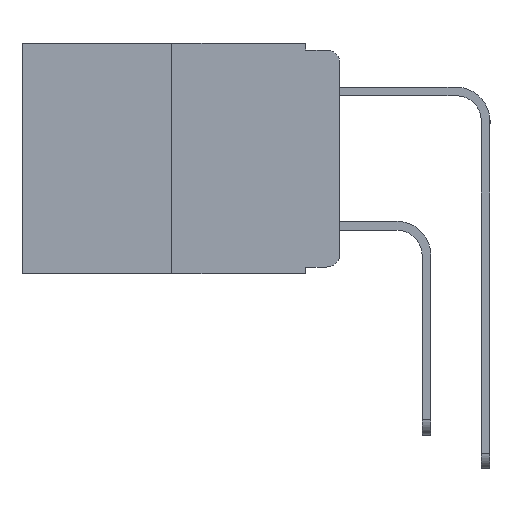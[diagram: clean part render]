
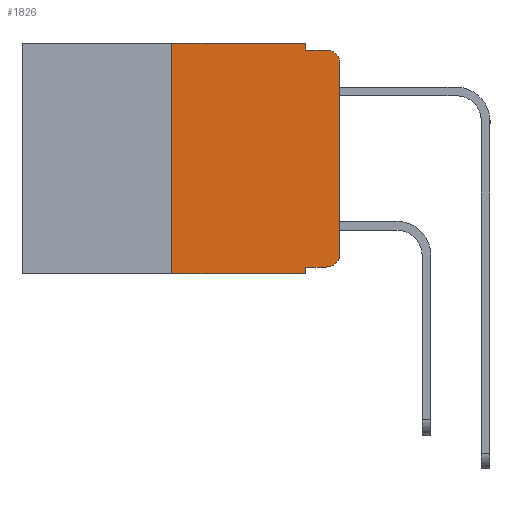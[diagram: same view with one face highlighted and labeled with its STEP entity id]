
A CAD part, left-side view. The second image highlights one B-rep face of the part: STEP entity #1826.
In plain terms, the highlighted planar face has unit normal (-1, 0, 0).
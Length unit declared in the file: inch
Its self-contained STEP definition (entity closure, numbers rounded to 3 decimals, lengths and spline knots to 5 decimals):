
#178 = FACE_OUTER_BOUND ( 'NONE', #17588, .T. ) ;
#365 = DIRECTION ( 'NONE',  ( 0., -1., 0. ) ) ;
#547 = VERTEX_POINT ( 'NONE', #4173 ) ;
#1144 = DIRECTION ( 'NONE',  ( 0., -1., 0. ) ) ;
#1159 = CARTESIAN_POINT ( 'NONE',  ( 0., 0., 0. ) ) ;
#1238 = EDGE_CURVE ( 'NONE', #547, #10272, #10835, .T. ) ;
#1810 = AXIS2_PLACEMENT_3D ( 'NONE', #14146, #5944, #15483 ) ;
#1826 = ADVANCED_FACE ( 'NONE', ( #178 ), #17150, .F. ) ;
#2052 = LINE ( 'NONE', #4103, #12909 ) ;
#3402 = DIRECTION ( 'NONE',  ( 0., 0., -1. ) ) ;
#3408 = VERTEX_POINT ( 'NONE', #6793 ) ;
#3584 = VERTEX_POINT ( 'NONE', #5995 ) ;
#3617 = EDGE_CURVE ( 'NONE', #3408, #16759, #14103, .T. ) ;
#3671 = ORIENTED_EDGE ( 'NONE', *, *, #1238, .F. ) ;
#3751 = AXIS2_PLACEMENT_3D ( 'NONE', #17131, #18101, #16671 ) ;
#3930 = AXIS2_PLACEMENT_3D ( 'NONE', #8382, #17770, #9779 ) ;
#4103 = CARTESIAN_POINT ( 'NONE',  ( 0., 0.051, 0. ) ) ;
#4173 = CARTESIAN_POINT ( 'NONE',  ( 0., 0.051, -0.01 ) ) ;
#4498 = DIRECTION ( 'NONE',  ( 0., -1., 0. ) ) ;
#4552 = VERTEX_POINT ( 'NONE', #11109 ) ;
#4815 = CARTESIAN_POINT ( 'NONE',  ( 0., 0.051, -0.01 ) ) ;
#4975 = CARTESIAN_POINT ( 'NONE',  ( 0., 0.051, -0.333 ) ) ;
#5243 = EDGE_CURVE ( 'NONE', #13959, #10272, #8101, .T. ) ;
#5551 = LINE ( 'NONE', #9230, #15588 ) ;
#5595 = DIRECTION ( 'NONE',  ( 0., 0., -1. ) ) ;
#5944 = DIRECTION ( 'NONE',  ( -1., 0., 0. ) ) ;
#5995 = CARTESIAN_POINT ( 'NONE',  ( 0., 0.25, 0. ) ) ;
#6417 = VECTOR ( 'NONE', #1144, 39.37008 ) ;
#6580 = ORIENTED_EDGE ( 'NONE', *, *, #5243, .T. ) ;
#6598 = ORIENTED_EDGE ( 'NONE', *, *, #8454, .T. ) ;
#6631 = ORIENTED_EDGE ( 'NONE', *, *, #10300, .T. ) ;
#6708 = VECTOR ( 'NONE', #4498, 39.37008 ) ;
#6731 = LINE ( 'NONE', #15886, #11270 ) ;
#6792 = DIRECTION ( 'NONE',  ( 0., 0., 1. ) ) ;
#6793 = CARTESIAN_POINT ( 'NONE',  ( 0., 0.25, -0.343 ) ) ;
#6950 = ORIENTED_EDGE ( 'NONE', *, *, #12115, .F. ) ;
#6985 = ORIENTED_EDGE ( 'NONE', *, *, #3617, .T. ) ;
#7147 = EDGE_CURVE ( 'NONE', #12108, #13959, #9990, .T. ) ;
#7496 = LINE ( 'NONE', #13595, #10765 ) ;
#8101 = CIRCLE ( 'NONE', #3930, 0.02 ) ;
#8382 = CARTESIAN_POINT ( 'NONE',  ( 0., 0.02, -0.03 ) ) ;
#8406 = VECTOR ( 'NONE', #365, 39.37008 ) ;
#8454 = EDGE_CURVE ( 'NONE', #4552, #12108, #13535, .T. ) ;
#8632 = ORIENTED_EDGE ( 'NONE', *, *, #9166, .F. ) ;
#8663 = VERTEX_POINT ( 'NONE', #4975 ) ;
#9166 = EDGE_CURVE ( 'NONE', #3584, #10078, #5551, .T. ) ;
#9230 = CARTESIAN_POINT ( 'NONE',  ( 0., 0.473, 0. ) ) ;
#9309 = ORIENTED_EDGE ( 'NONE', *, *, #17439, .F. ) ;
#9779 = DIRECTION ( 'NONE',  ( 0., 0., -1. ) ) ;
#9990 = LINE ( 'NONE', #1159, #13569 ) ;
#10078 = VERTEX_POINT ( 'NONE', #14030 ) ;
#10272 = VERTEX_POINT ( 'NONE', #14428 ) ;
#10300 = EDGE_CURVE ( 'NONE', #8663, #4552, #11600, .T. ) ;
#10518 = CARTESIAN_POINT ( 'NONE',  ( 0., 0., -0.03 ) ) ;
#10765 = VECTOR ( 'NONE', #6792, 39.37008 ) ;
#10835 = LINE ( 'NONE', #4815, #6708 ) ;
#11109 = CARTESIAN_POINT ( 'NONE',  ( 0., 0.02, -0.333 ) ) ;
#11188 = DIRECTION ( 'NONE',  ( 0., 0., 1. ) ) ;
#11270 = VECTOR ( 'NONE', #3402, 39.37008 ) ;
#11600 = LINE ( 'NONE', #17156, #8406 ) ;
#12108 = VERTEX_POINT ( 'NONE', #17158 ) ;
#12115 = EDGE_CURVE ( 'NONE', #8663, #16759, #6731, .T. ) ;
#12909 = VECTOR ( 'NONE', #5595, 39.37008 ) ;
#13535 = CIRCLE ( 'NONE', #1810, 0.02 ) ;
#13569 = VECTOR ( 'NONE', #11188, 39.37008 ) ;
#13595 = CARTESIAN_POINT ( 'NONE',  ( 0., 0.25, 0. ) ) ;
#13959 = VERTEX_POINT ( 'NONE', #10518 ) ;
#14030 = CARTESIAN_POINT ( 'NONE',  ( 0., 0.051, 0. ) ) ;
#14103 = LINE ( 'NONE', #15874, #6417 ) ;
#14146 = CARTESIAN_POINT ( 'NONE',  ( 0., 0.02, -0.313 ) ) ;
#14428 = CARTESIAN_POINT ( 'NONE',  ( 0., 0.02, -0.01 ) ) ;
#14789 = EDGE_CURVE ( 'NONE', #3408, #3584, #7496, .T. ) ;
#15002 = ORIENTED_EDGE ( 'NONE', *, *, #14789, .F. ) ;
#15072 = CARTESIAN_POINT ( 'NONE',  ( 0., 0.051, -0.343 ) ) ;
#15483 = DIRECTION ( 'NONE',  ( 0., 0., -1. ) ) ;
#15588 = VECTOR ( 'NONE', #17262, 39.37008 ) ;
#15867 = ORIENTED_EDGE ( 'NONE', *, *, #7147, .T. ) ;
#15874 = CARTESIAN_POINT ( 'NONE',  ( 0., 0.473, -0.343 ) ) ;
#15886 = CARTESIAN_POINT ( 'NONE',  ( 0., 0.051, 0. ) ) ;
#16671 = DIRECTION ( 'NONE',  ( 0., 0., -1. ) ) ;
#16759 = VERTEX_POINT ( 'NONE', #15072 ) ;
#17131 = CARTESIAN_POINT ( 'NONE',  ( 0., 0.473, 0. ) ) ;
#17150 = PLANE ( 'NONE',  #3751 ) ;
#17156 = CARTESIAN_POINT ( 'NONE',  ( 0., 0.051, -0.333 ) ) ;
#17158 = CARTESIAN_POINT ( 'NONE',  ( 0., 0., -0.313 ) ) ;
#17262 = DIRECTION ( 'NONE',  ( 0., -1., 0. ) ) ;
#17439 = EDGE_CURVE ( 'NONE', #10078, #547, #2052, .T. ) ;
#17588 = EDGE_LOOP ( 'NONE', ( #15867, #6580, #3671, #9309, #8632, #15002, #6985, #6950, #6631, #6598 ) ) ;
#17770 = DIRECTION ( 'NONE',  ( -1., 0., 0. ) ) ;
#18101 = DIRECTION ( 'NONE',  ( 1., 0., 0. ) ) ;
